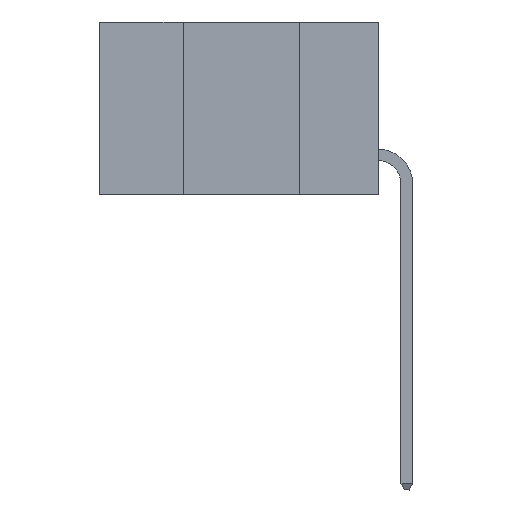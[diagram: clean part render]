
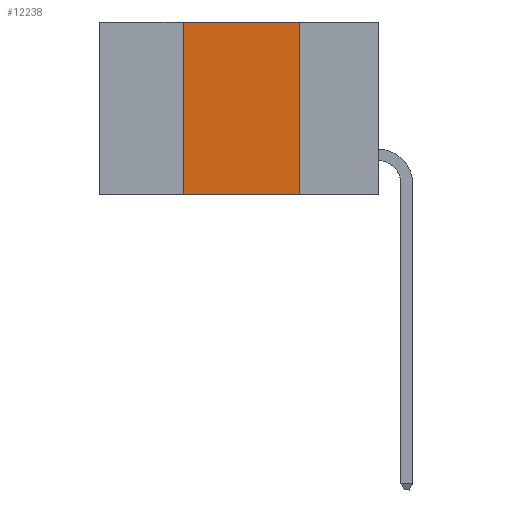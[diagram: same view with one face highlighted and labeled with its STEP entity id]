
A CAD part, left-side view. The second image highlights one B-rep face of the part: STEP entity #12238.
In plain terms, the highlighted planar face has unit normal (-1, 0, 0).
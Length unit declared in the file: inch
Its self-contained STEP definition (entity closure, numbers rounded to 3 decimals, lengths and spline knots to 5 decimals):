
#258 = EDGE_CURVE ( 'NONE', #10659, #14209, #8037, .T. ) ;
#777 = VERTEX_POINT ( 'NONE', #12068 ) ;
#1387 = DIRECTION ( 'NONE',  ( 0., 0., 1. ) ) ;
#1814 = LINE ( 'NONE', #6253, #4074 ) ;
#2276 = EDGE_CURVE ( 'NONE', #3255, #777, #1814, .T. ) ;
#2338 = CARTESIAN_POINT ( 'NONE',  ( 0., 0.6, 0. ) ) ;
#2537 = CARTESIAN_POINT ( 'NONE',  ( 0., 0.6, 0. ) ) ;
#2593 = DIRECTION ( 'NONE',  ( 0., 0., -1. ) ) ;
#3241 = CARTESIAN_POINT ( 'NONE',  ( 0., 0.17, 0. ) ) ;
#3255 = VERTEX_POINT ( 'NONE', #3241 ) ;
#3753 = VECTOR ( 'NONE', #5854, 39.37008 ) ;
#4074 = VECTOR ( 'NONE', #11114, 39.37008 ) ;
#4539 = ORIENTED_EDGE ( 'NONE', *, *, #10175, .T. ) ;
#5614 = ORIENTED_EDGE ( 'NONE', *, *, #2276, .F. ) ;
#5854 = DIRECTION ( 'NONE',  ( 0., -1., 0. ) ) ;
#6253 = CARTESIAN_POINT ( 'NONE',  ( 0., 0.17, 0. ) ) ;
#7458 = CARTESIAN_POINT ( 'NONE',  ( 0., 0.42, -0.37 ) ) ;
#8037 = LINE ( 'NONE', #10838, #12135 ) ;
#8441 = EDGE_LOOP ( 'NONE', ( #5614, #14802, #12702, #4539 ) ) ;
#8693 = CARTESIAN_POINT ( 'NONE',  ( 0., 0.6, -0.37 ) ) ;
#9082 = FACE_OUTER_BOUND ( 'NONE', #8441, .T. ) ;
#9124 = VECTOR ( 'NONE', #13666, 39.37008 ) ;
#9642 = PLANE ( 'NONE',  #11056 ) ;
#10175 = EDGE_CURVE ( 'NONE', #10659, #777, #10280, .T. ) ;
#10280 = LINE ( 'NONE', #8693, #9124 ) ;
#10659 = VERTEX_POINT ( 'NONE', #7458 ) ;
#10838 = CARTESIAN_POINT ( 'NONE',  ( 0., 0.42, 0. ) ) ;
#11056 = AXIS2_PLACEMENT_3D ( 'NONE', #2537, #12059, #2593 ) ;
#11114 = DIRECTION ( 'NONE',  ( 0., 0., -1. ) ) ;
#11309 = CARTESIAN_POINT ( 'NONE',  ( 0., 0.42, 0. ) ) ;
#11532 = EDGE_CURVE ( 'NONE', #14209, #3255, #14733, .T. ) ;
#12059 = DIRECTION ( 'NONE',  ( 1., 0., 0. ) ) ;
#12068 = CARTESIAN_POINT ( 'NONE',  ( 0., 0.17, -0.37 ) ) ;
#12135 = VECTOR ( 'NONE', #1387, 39.37008 ) ;
#12238 = ADVANCED_FACE ( 'NONE', ( #9082 ), #9642, .F. ) ;
#12702 = ORIENTED_EDGE ( 'NONE', *, *, #258, .F. ) ;
#13666 = DIRECTION ( 'NONE',  ( 0., -1., 0. ) ) ;
#14209 = VERTEX_POINT ( 'NONE', #11309 ) ;
#14733 = LINE ( 'NONE', #2338, #3753 ) ;
#14802 = ORIENTED_EDGE ( 'NONE', *, *, #11532, .F. ) ;
